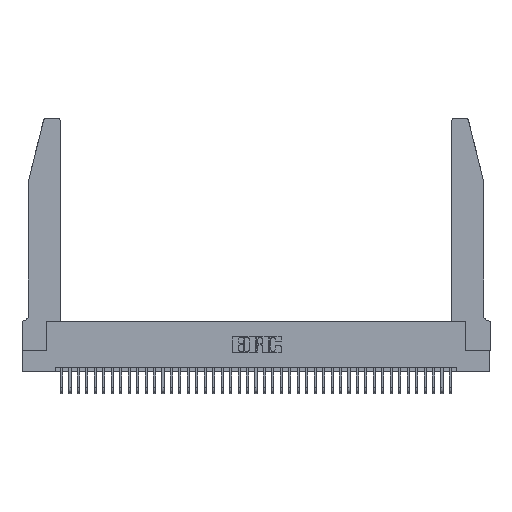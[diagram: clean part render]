
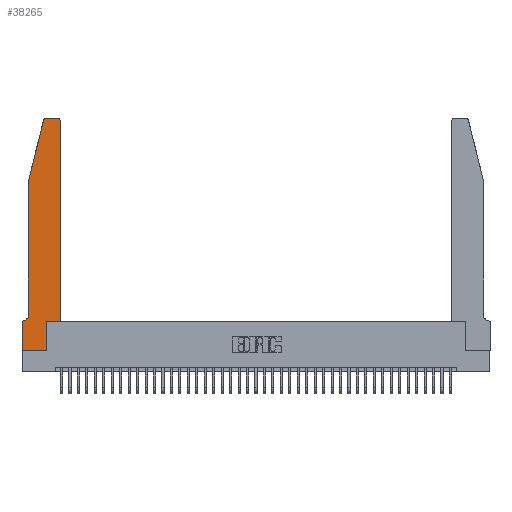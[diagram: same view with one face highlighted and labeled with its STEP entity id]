
A CAD part, top view. The second image highlights one B-rep face of the part: STEP entity #38265.
In plain terms, the highlighted planar face has unit normal (0, 0, 1).
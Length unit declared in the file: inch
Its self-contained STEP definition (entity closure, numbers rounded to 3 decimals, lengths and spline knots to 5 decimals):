
#318 = DIRECTION ( 'NONE',  ( 0., 0., 1. ) ) ;
#610 = EDGE_CURVE ( 'NONE', #994, #18194, #3717, .T. ) ;
#682 = VECTOR ( 'NONE', #16758, 39.37008 ) ;
#700 = CARTESIAN_POINT ( 'NONE',  ( 0., 0.35, 0.37 ) ) ;
#763 = VECTOR ( 'NONE', #20793, 39.37008 ) ;
#994 = VERTEX_POINT ( 'NONE', #4422 ) ;
#1362 = ORIENTED_EDGE ( 'NONE', *, *, #26299, .T. ) ;
#1613 = VECTOR ( 'NONE', #30469, 39.37008 ) ;
#1670 = VERTEX_POINT ( 'NONE', #4508 ) ;
#3391 = CARTESIAN_POINT ( 'NONE',  ( 0.0755, 2., 0.37 ) ) ;
#3418 = AXIS2_PLACEMENT_3D ( 'NONE', #18743, #318, #21794 ) ;
#3637 = ORIENTED_EDGE ( 'NONE', *, *, #29925, .T. ) ;
#3717 = LINE ( 'NONE', #33125, #35233 ) ;
#4422 = CARTESIAN_POINT ( 'NONE',  ( 0., 0., 0.37 ) ) ;
#4508 = CARTESIAN_POINT ( 'NONE',  ( 0.25487, 2.72718, 0.37 ) ) ;
#4841 = EDGE_CURVE ( 'NONE', #5474, #33900, #31977, .T. ) ;
#5474 = VERTEX_POINT ( 'NONE', #18469 ) ;
#5550 = CIRCLE ( 'NONE', #7069, 0.03 ) ;
#6088 = VERTEX_POINT ( 'NONE', #3391 ) ;
#6212 = EDGE_CURVE ( 'NONE', #17862, #1670, #5550, .T. ) ;
#7032 = DIRECTION ( 'NONE',  ( 0., 0., 1. ) ) ;
#7069 = AXIS2_PLACEMENT_3D ( 'NONE', #13339, #34611, #16430 ) ;
#7960 = VERTEX_POINT ( 'NONE', #18813 ) ;
#8026 = LINE ( 'NONE', #38941, #763 ) ;
#8060 = CARTESIAN_POINT ( 'NONE',  ( 0.0755, 2., 0.37 ) ) ;
#8109 = ORIENTED_EDGE ( 'NONE', *, *, #18965, .T. ) ;
#9272 = VECTOR ( 'NONE', #34934, 39.37008 ) ;
#9763 = LINE ( 'NONE', #39436, #1613 ) ;
#9867 = DIRECTION ( 'NONE',  ( 0., 1., 0. ) ) ;
#10307 = EDGE_CURVE ( 'NONE', #6088, #10952, #8026, .T. ) ;
#10326 = ORIENTED_EDGE ( 'NONE', *, *, #6212, .T. ) ;
#10952 = VERTEX_POINT ( 'NONE', #11961 ) ;
#11315 = ORIENTED_EDGE ( 'NONE', *, *, #21076, .T. ) ;
#11624 = AXIS2_PLACEMENT_3D ( 'NONE', #12950, #34207, #16022 ) ;
#11842 = DIRECTION ( 'NONE',  ( 1., 0., 0. ) ) ;
#11961 = CARTESIAN_POINT ( 'NONE',  ( 0.0755, 0.42, 0.37 ) ) ;
#12508 = VECTOR ( 'NONE', #26368, 39.37008 ) ;
#12815 = CARTESIAN_POINT ( 'NONE',  ( 0.4505, 0.35, 0.37 ) ) ;
#12886 = CARTESIAN_POINT ( 'NONE',  ( 0.0055, 0.35, 0.37 ) ) ;
#12950 = CARTESIAN_POINT ( 'NONE',  ( 0.0055, 0.42, 0.37 ) ) ;
#13339 = CARTESIAN_POINT ( 'NONE',  ( 0.284, 2.72, 0.37 ) ) ;
#13478 = LINE ( 'NONE', #8060, #12508 ) ;
#13538 = CARTESIAN_POINT ( 'NONE',  ( 0., 0., 0.37 ) ) ;
#13803 = CARTESIAN_POINT ( 'NONE',  ( 0.0755, 0.35, 0.37 ) ) ;
#14926 = FACE_OUTER_BOUND ( 'NONE', #39074, .T. ) ;
#16022 = DIRECTION ( 'NONE',  ( -1., 0., 0. ) ) ;
#16430 = DIRECTION ( 'NONE',  ( 1., 0., 0. ) ) ;
#16480 = VECTOR ( 'NONE', #28402, 39.37008 ) ;
#16519 = LINE ( 'NONE', #13538, #9272 ) ;
#16758 = DIRECTION ( 'NONE',  ( -1., 0., 0. ) ) ;
#17862 = VERTEX_POINT ( 'NONE', #35651 ) ;
#18146 = CARTESIAN_POINT ( 'NONE',  ( 0.4505, 0.35, 0.37 ) ) ;
#18194 = VERTEX_POINT ( 'NONE', #22093 ) ;
#18277 = DIRECTION ( 'NONE',  ( 0., 1., 0. ) ) ;
#18337 = LINE ( 'NONE', #18146, #19294 ) ;
#18344 = CARTESIAN_POINT ( 'NONE',  ( 0.2865, 0.35, 0.37 ) ) ;
#18469 = CARTESIAN_POINT ( 'NONE',  ( 0.4505, 2.72, 0.37 ) ) ;
#18743 = CARTESIAN_POINT ( 'NONE',  ( 0.4205, 2.72, 0.37 ) ) ;
#18813 = CARTESIAN_POINT ( 'NONE',  ( 0., 0.35, 0.37 ) ) ;
#18947 = ORIENTED_EDGE ( 'NONE', *, *, #36922, .T. ) ;
#18965 = EDGE_CURVE ( 'NONE', #32533, #7960, #23259, .T. ) ;
#19294 = VECTOR ( 'NONE', #18277, 39.37008 ) ;
#19765 = EDGE_CURVE ( 'NONE', #23959, #28520, #9763, .T. ) ;
#20793 = DIRECTION ( 'NONE',  ( 0., -1., 0. ) ) ;
#21076 = EDGE_CURVE ( 'NONE', #28520, #5474, #18337, .T. ) ;
#21794 = DIRECTION ( 'NONE',  ( 1., 0., 0. ) ) ;
#22093 = CARTESIAN_POINT ( 'NONE',  ( 0.2865, 0., 0.37 ) ) ;
#22430 = EDGE_CURVE ( 'NONE', #18194, #23959, #25389, .T. ) ;
#22968 = CIRCLE ( 'NONE', #11624, 0.07 ) ;
#23259 = LINE ( 'NONE', #13803, #682 ) ;
#23959 = VERTEX_POINT ( 'NONE', #18344 ) ;
#24947 = AXIS2_PLACEMENT_3D ( 'NONE', #700, #7032, #28430 ) ;
#25388 = PLANE ( 'NONE',  #24947 ) ;
#25389 = LINE ( 'NONE', #37005, #32500 ) ;
#26299 = EDGE_CURVE ( 'NONE', #1670, #6088, #13478, .T. ) ;
#26368 = DIRECTION ( 'NONE',  ( -0.239, -0.971, 0. ) ) ;
#27490 = ORIENTED_EDGE ( 'NONE', *, *, #30378, .T. ) ;
#28010 = ORIENTED_EDGE ( 'NONE', *, *, #19765, .T. ) ;
#28402 = DIRECTION ( 'NONE',  ( -1., 0., 0. ) ) ;
#28430 = DIRECTION ( 'NONE',  ( 1., 0., 0. ) ) ;
#28520 = VERTEX_POINT ( 'NONE', #12815 ) ;
#29925 = EDGE_CURVE ( 'NONE', #7960, #994, #16519, .T. ) ;
#30106 = ORIENTED_EDGE ( 'NONE', *, *, #10307, .T. ) ;
#30378 = EDGE_CURVE ( 'NONE', #33900, #17862, #31679, .T. ) ;
#30469 = DIRECTION ( 'NONE',  ( 1., 0., 0. ) ) ;
#31448 = CARTESIAN_POINT ( 'NONE',  ( 0.2605, 2.75, 0.37 ) ) ;
#31679 = LINE ( 'NONE', #31448, #16480 ) ;
#31779 = ORIENTED_EDGE ( 'NONE', *, *, #22430, .T. ) ;
#31977 = CIRCLE ( 'NONE', #3418, 0.03 ) ;
#32500 = VECTOR ( 'NONE', #9867, 39.37008 ) ;
#32502 = ORIENTED_EDGE ( 'NONE', *, *, #610, .T. ) ;
#32533 = VERTEX_POINT ( 'NONE', #12886 ) ;
#33125 = CARTESIAN_POINT ( 'NONE',  ( 0., 0., 0.37 ) ) ;
#33481 = CARTESIAN_POINT ( 'NONE',  ( 0.4205, 2.75, 0.37 ) ) ;
#33900 = VERTEX_POINT ( 'NONE', #33481 ) ;
#34207 = DIRECTION ( 'NONE',  ( 0., 0., -1. ) ) ;
#34611 = DIRECTION ( 'NONE',  ( 0., 0., 1. ) ) ;
#34934 = DIRECTION ( 'NONE',  ( 0., -1., 0. ) ) ;
#35233 = VECTOR ( 'NONE', #11842, 39.37008 ) ;
#35651 = CARTESIAN_POINT ( 'NONE',  ( 0.284, 2.75, 0.37 ) ) ;
#36922 = EDGE_CURVE ( 'NONE', #10952, #32533, #22968, .T. ) ;
#37005 = CARTESIAN_POINT ( 'NONE',  ( 0.2865, 0.35, 0.37 ) ) ;
#38210 = ORIENTED_EDGE ( 'NONE', *, *, #4841, .T. ) ;
#38265 = ADVANCED_FACE ( 'NONE', ( #14926 ), #25388, .T. ) ;
#38941 = CARTESIAN_POINT ( 'NONE',  ( 0.0755, 2., 0.37 ) ) ;
#39074 = EDGE_LOOP ( 'NONE', ( #27490, #10326, #1362, #30106, #18947, #8109, #3637, #32502, #31779, #28010, #11315, #38210 ) ) ;
#39436 = CARTESIAN_POINT ( 'NONE',  ( 0.4505, 0.35, 0.37 ) ) ;
